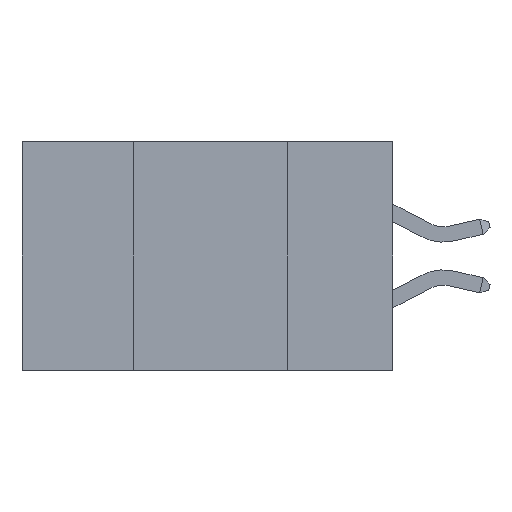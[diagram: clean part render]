
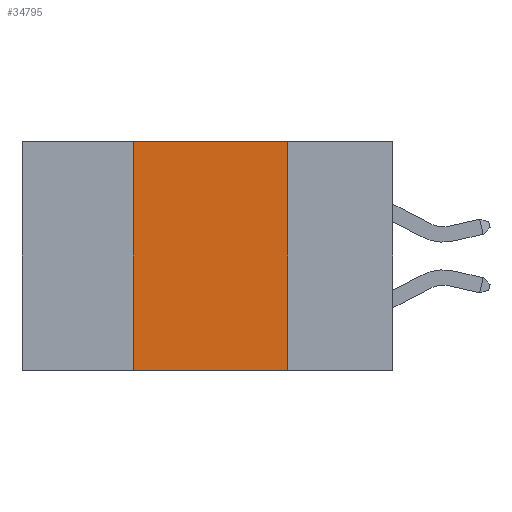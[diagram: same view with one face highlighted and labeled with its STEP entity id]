
A CAD part, left-side view. The second image highlights one B-rep face of the part: STEP entity #34795.
In plain terms, the highlighted planar face has unit normal (-1, 0, 0).
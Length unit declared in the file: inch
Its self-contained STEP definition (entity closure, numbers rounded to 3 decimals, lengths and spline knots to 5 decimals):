
#67 = CARTESIAN_POINT ( 'NONE',  ( 0., 0.17, 0. ) ) ;
#638 = CARTESIAN_POINT ( 'NONE',  ( 0., 0.17, -0.37 ) ) ;
#1030 = DIRECTION ( 'NONE',  ( 0., -1., 0. ) ) ;
#1935 = EDGE_CURVE ( 'NONE', #2358, #16962, #29471, .T. ) ;
#2358 = VERTEX_POINT ( 'NONE', #4399 ) ;
#2528 = DIRECTION ( 'NONE',  ( 0., 0., 1. ) ) ;
#3160 = EDGE_CURVE ( 'NONE', #2358, #11867, #13999, .T. ) ;
#3343 = DIRECTION ( 'NONE',  ( 1., 0., 0. ) ) ;
#4135 = VERTEX_POINT ( 'NONE', #67 ) ;
#4233 = DIRECTION ( 'NONE',  ( 0., -1., 0. ) ) ;
#4399 = CARTESIAN_POINT ( 'NONE',  ( 0., 0.42, -0.37 ) ) ;
#5315 = LINE ( 'NONE', #34752, #20310 ) ;
#5655 = VECTOR ( 'NONE', #4233, 39.37008 ) ;
#5798 = FACE_OUTER_BOUND ( 'NONE', #12411, .T. ) ;
#7023 = VECTOR ( 'NONE', #27260, 39.37008 ) ;
#10816 = ORIENTED_EDGE ( 'NONE', *, *, #1935, .F. ) ;
#10939 = CARTESIAN_POINT ( 'NONE',  ( 0., 0.42, 0. ) ) ;
#11867 = VERTEX_POINT ( 'NONE', #638 ) ;
#12411 = EDGE_LOOP ( 'NONE', ( #13906, #32343, #10816, #13472 ) ) ;
#13237 = CARTESIAN_POINT ( 'NONE',  ( 0., 0.17, 0. ) ) ;
#13472 = ORIENTED_EDGE ( 'NONE', *, *, #3160, .T. ) ;
#13906 = ORIENTED_EDGE ( 'NONE', *, *, #35771, .F. ) ;
#13999 = LINE ( 'NONE', #23938, #5655 ) ;
#14435 = PLANE ( 'NONE',  #35054 ) ;
#16300 = VECTOR ( 'NONE', #2528, 39.37008 ) ;
#16962 = VERTEX_POINT ( 'NONE', #10939 ) ;
#20310 = VECTOR ( 'NONE', #1030, 39.37008 ) ;
#23047 = DIRECTION ( 'NONE',  ( 0., 0., -1. ) ) ;
#23775 = LINE ( 'NONE', #13237, #7023 ) ;
#23884 = EDGE_CURVE ( 'NONE', #16962, #4135, #5315, .T. ) ;
#23938 = CARTESIAN_POINT ( 'NONE',  ( 0., 0.6, -0.37 ) ) ;
#27260 = DIRECTION ( 'NONE',  ( 0., 0., -1. ) ) ;
#29471 = LINE ( 'NONE', #36107, #16300 ) ;
#32343 = ORIENTED_EDGE ( 'NONE', *, *, #23884, .F. ) ;
#34157 = CARTESIAN_POINT ( 'NONE',  ( 0., 0.6, 0. ) ) ;
#34752 = CARTESIAN_POINT ( 'NONE',  ( 0., 0.6, 0. ) ) ;
#34795 = ADVANCED_FACE ( 'NONE', ( #5798 ), #14435, .F. ) ;
#35054 = AXIS2_PLACEMENT_3D ( 'NONE', #34157, #3343, #23047 ) ;
#35771 = EDGE_CURVE ( 'NONE', #4135, #11867, #23775, .T. ) ;
#36107 = CARTESIAN_POINT ( 'NONE',  ( 0., 0.42, 0. ) ) ;
